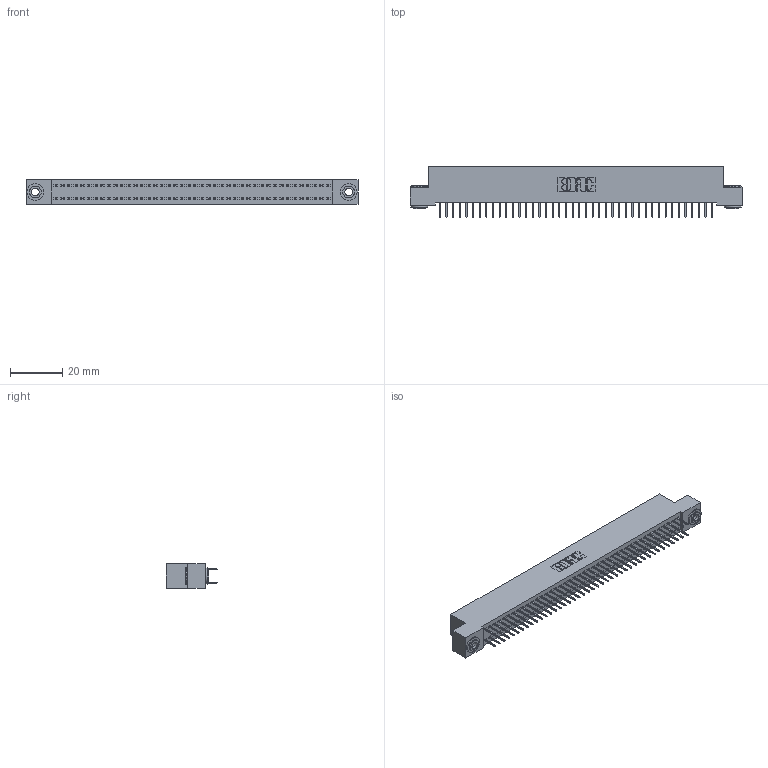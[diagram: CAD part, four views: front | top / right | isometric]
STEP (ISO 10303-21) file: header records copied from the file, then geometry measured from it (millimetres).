
FILE_DESCRIPTION (( 'STEP AP203' ), '1' );
FILE_NAME ('392-084-524-203.STEP', '2019-10-09T15:33:39', ( '' ), ( '' ), 'SwSTEP 2.0', 'SolidWorks 2016', '' );
FILE_SCHEMA (( 'CONFIG_CONTROL_DESIGN' ));
Length unit declared in the file: inch
Products named in the file (4): 342 Part_.156 TH; 345-292-001_345-293-124; 342-250-002_345-250-002-102; 392-084-524-203
Assembly tree (87 placements, depth 2):
  392-084-524-203
    342 Part_.156 TH
    345-292-001_345-293-124  x84
    342-250-002_345-250-002-102  x2
Bounding box: 127 x 19.69 x 9.4 mm (x, y, z)
Volume: 11306.6 mm3; surface area: 18287.8 mm2
Topology: 87 solids, 87 shells, 4852 faces, 13731 edges, 8814 vertices
Faces by surface type: plane 3604, cylinder 1240, cone 8
Entity records: 27612 total; most frequent: CARTESIAN_POINT 4549, ORIENTED_EDGE 4478, DIRECTION 3921, EDGE_CURVE 2239, VECTOR 2091, LINE 2091, VERTEX_POINT 1486, AXIS2_PLACEMENT_3D 915
